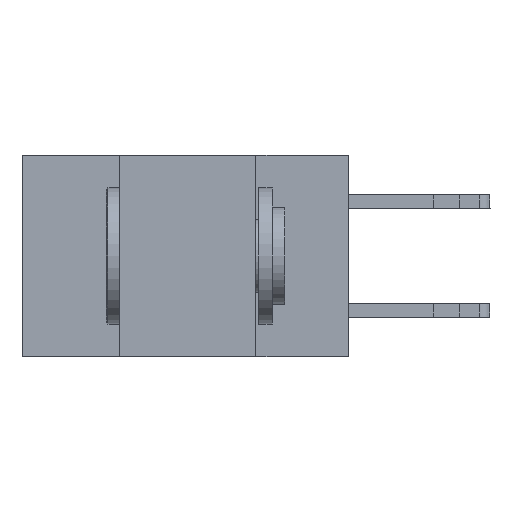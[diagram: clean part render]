
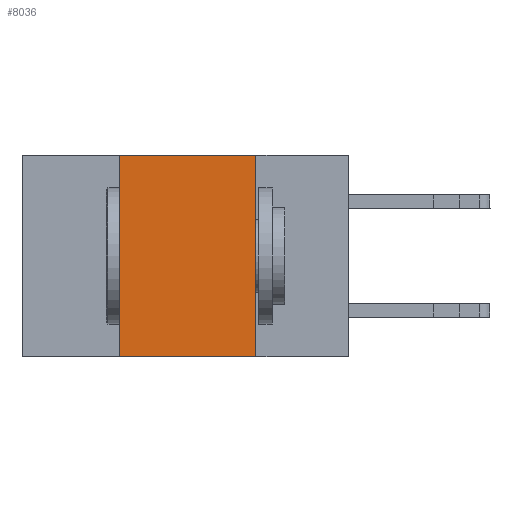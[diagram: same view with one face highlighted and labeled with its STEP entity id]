
A CAD part, left-side view. The second image highlights one B-rep face of the part: STEP entity #8036.
In plain terms, the highlighted planar face has unit normal (-1, 0, 0).
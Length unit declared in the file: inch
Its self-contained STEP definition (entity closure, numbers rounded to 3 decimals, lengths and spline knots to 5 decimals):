
#1402 = CARTESIAN_POINT ( 'NONE',  ( 0., 0.42, -0.37 ) ) ;
#1417 = DIRECTION ( 'NONE',  ( 0., 0., -1. ) ) ;
#1601 = VECTOR ( 'NONE', #7400, 39.37008 ) ;
#1758 = EDGE_LOOP ( 'NONE', ( #9064, #13004, #7821, #18184 ) ) ;
#1937 = CARTESIAN_POINT ( 'NONE',  ( 0., 0.42, 0. ) ) ;
#2414 = VERTEX_POINT ( 'NONE', #12304 ) ;
#2434 = CARTESIAN_POINT ( 'NONE',  ( 0., 0.6, -0.37 ) ) ;
#3328 = VERTEX_POINT ( 'NONE', #16111 ) ;
#4483 = LINE ( 'NONE', #1402, #5589 ) ;
#5589 = VECTOR ( 'NONE', #9119, 39.37008 ) ;
#6116 = DIRECTION ( 'NONE',  ( 0., -1., 0. ) ) ;
#6325 = EDGE_CURVE ( 'NONE', #2414, #10447, #4483, .T. ) ;
#6596 = LINE ( 'NONE', #2434, #12987 ) ;
#7400 = DIRECTION ( 'NONE',  ( 0., 0., -1. ) ) ;
#7821 = ORIENTED_EDGE ( 'NONE', *, *, #6325, .F. ) ;
#8036 = ADVANCED_FACE ( 'NONE', ( #11904 ), #10423, .F. ) ;
#8797 = CARTESIAN_POINT ( 'NONE',  ( 0., 0.17, -0.37 ) ) ;
#9064 = ORIENTED_EDGE ( 'NONE', *, *, #12831, .F. ) ;
#9119 = DIRECTION ( 'NONE',  ( 0., 0., 1. ) ) ;
#10423 = PLANE ( 'NONE',  #12293 ) ;
#10447 = VERTEX_POINT ( 'NONE', #1937 ) ;
#10945 = CARTESIAN_POINT ( 'NONE',  ( 0., 0.6, 0. ) ) ;
#11870 = LINE ( 'NONE', #8797, #1601 ) ;
#11904 = FACE_OUTER_BOUND ( 'NONE', #1758, .T. ) ;
#12293 = AXIS2_PLACEMENT_3D ( 'NONE', #16246, #18130, #1417 ) ;
#12304 = CARTESIAN_POINT ( 'NONE',  ( 0., 0.42, -0.37 ) ) ;
#12813 = DIRECTION ( 'NONE',  ( 0., -1., 0. ) ) ;
#12831 = EDGE_CURVE ( 'NONE', #18098, #3328, #11870, .T. ) ;
#12987 = VECTOR ( 'NONE', #12813, 39.37008 ) ;
#13004 = ORIENTED_EDGE ( 'NONE', *, *, #13390, .F. ) ;
#13390 = EDGE_CURVE ( 'NONE', #10447, #18098, #18374, .T. ) ;
#13652 = EDGE_CURVE ( 'NONE', #2414, #3328, #6596, .T. ) ;
#15166 = VECTOR ( 'NONE', #6116, 39.37008 ) ;
#16111 = CARTESIAN_POINT ( 'NONE',  ( 0., 0.17, -0.37 ) ) ;
#16246 = CARTESIAN_POINT ( 'NONE',  ( 0., 0.6, 0. ) ) ;
#16500 = CARTESIAN_POINT ( 'NONE',  ( 0., 0.17, 0. ) ) ;
#18098 = VERTEX_POINT ( 'NONE', #16500 ) ;
#18130 = DIRECTION ( 'NONE',  ( 1., 0., 0. ) ) ;
#18184 = ORIENTED_EDGE ( 'NONE', *, *, #13652, .T. ) ;
#18374 = LINE ( 'NONE', #10945, #15166 ) ;
